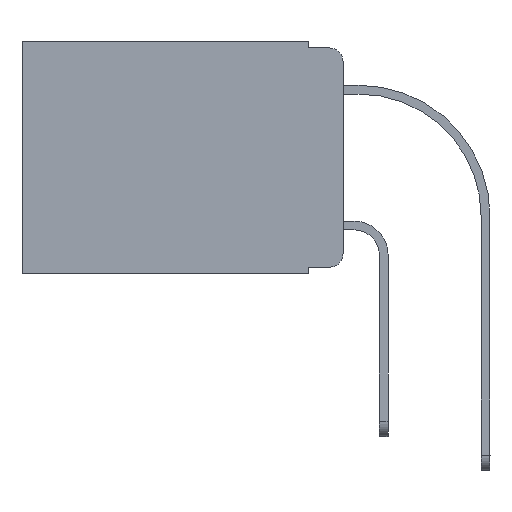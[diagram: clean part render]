
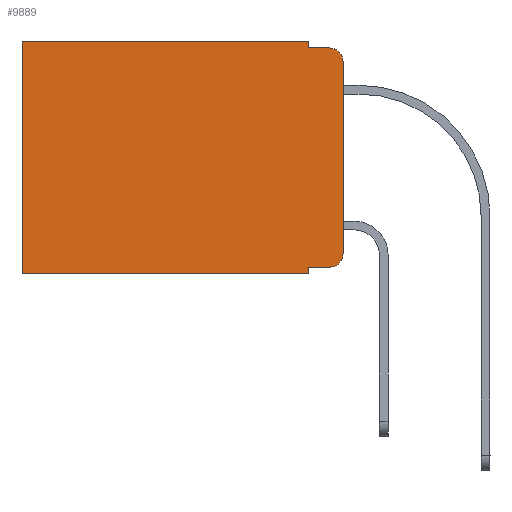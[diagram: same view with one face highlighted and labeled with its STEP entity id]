
A CAD part, left-side view. The second image highlights one B-rep face of the part: STEP entity #9889.
In plain terms, the highlighted planar face has unit normal (-1, 0, 0).
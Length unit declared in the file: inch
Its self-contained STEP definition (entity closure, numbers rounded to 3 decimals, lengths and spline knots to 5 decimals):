
#12 = CIRCLE ( 'NONE', #15573, 0.02 ) ;
#276 = ORIENTED_EDGE ( 'NONE', *, *, #1534, .F. ) ;
#453 = ORIENTED_EDGE ( 'NONE', *, *, #14678, .F. ) ;
#655 = CARTESIAN_POINT ( 'NONE',  ( 0.298, 0.02, -0.03 ) ) ;
#703 = VERTEX_POINT ( 'NONE', #19091 ) ;
#800 = DIRECTION ( 'NONE',  ( -1., 0., 0. ) ) ;
#911 = CARTESIAN_POINT ( 'NONE',  ( 0.298, 0., 0. ) ) ;
#935 = CARTESIAN_POINT ( 'NONE',  ( 0.298, 0.051, 0. ) ) ;
#1233 = DIRECTION ( 'NONE',  ( 1., 0., 0. ) ) ;
#1250 = LINE ( 'NONE', #10990, #7418 ) ;
#1534 = EDGE_CURVE ( 'NONE', #19817, #13339, #12464, .T. ) ;
#2334 = DIRECTION ( 'NONE',  ( 0., 0., -1. ) ) ;
#2341 = ORIENTED_EDGE ( 'NONE', *, *, #10339, .T. ) ;
#2630 = DIRECTION ( 'NONE',  ( 0., 0., -1. ) ) ;
#3657 = ORIENTED_EDGE ( 'NONE', *, *, #18781, .F. ) ;
#3850 = ORIENTED_EDGE ( 'NONE', *, *, #15713, .T. ) ;
#4126 = VERTEX_POINT ( 'NONE', #8880 ) ;
#4248 = VERTEX_POINT ( 'NONE', #20828 ) ;
#5466 = CARTESIAN_POINT ( 'NONE',  ( 0.298, 0.051, -0.01 ) ) ;
#6257 = CARTESIAN_POINT ( 'NONE',  ( 0.298, 0.051, -0.01 ) ) ;
#6722 = EDGE_CURVE ( 'NONE', #4126, #6739, #8010, .T. ) ;
#6739 = VERTEX_POINT ( 'NONE', #15595 ) ;
#6804 = LINE ( 'NONE', #13262, #10517 ) ;
#6893 = CARTESIAN_POINT ( 'NONE',  ( 0.298, 0.051, -0.333 ) ) ;
#7125 = DIRECTION ( 'NONE',  ( -1., 0., 0. ) ) ;
#7368 = DIRECTION ( 'NONE',  ( 0., 1., 0. ) ) ;
#7418 = VECTOR ( 'NONE', #2630, 39.37008 ) ;
#8010 = CIRCLE ( 'NONE', #11378, 0.02 ) ;
#8128 = CARTESIAN_POINT ( 'NONE',  ( 0.298, 0.02, -0.333 ) ) ;
#8704 = EDGE_LOOP ( 'NONE', ( #453, #10495, #18752, #3657, #20559, #9937, #276, #16006, #3850, #2341 ) ) ;
#8880 = CARTESIAN_POINT ( 'NONE',  ( 0.298, 0., -0.03 ) ) ;
#8945 = CARTESIAN_POINT ( 'NONE',  ( 0.298, 0.02, -0.313 ) ) ;
#9062 = DIRECTION ( 'NONE',  ( 0., 0., -1. ) ) ;
#9746 = VERTEX_POINT ( 'NONE', #8128 ) ;
#9889 = ADVANCED_FACE ( 'NONE', ( #12550 ), #12346, .F. ) ;
#9937 = ORIENTED_EDGE ( 'NONE', *, *, #14060, .T. ) ;
#10339 = EDGE_CURVE ( 'NONE', #9746, #703, #12, .T. ) ;
#10361 = DIRECTION ( 'NONE',  ( 0., 0., -1. ) ) ;
#10495 = ORIENTED_EDGE ( 'NONE', *, *, #6722, .T. ) ;
#10517 = VECTOR ( 'NONE', #19412, 39.37008 ) ;
#10990 = CARTESIAN_POINT ( 'NONE',  ( 0.298, 0.051, 0. ) ) ;
#11378 = AXIS2_PLACEMENT_3D ( 'NONE', #655, #7125, #15162 ) ;
#12094 = CARTESIAN_POINT ( 'NONE',  ( 0.298, 0.473, 0. ) ) ;
#12346 = PLANE ( 'NONE',  #15876 ) ;
#12443 = CARTESIAN_POINT ( 'NONE',  ( 0.298, 0., 0. ) ) ;
#12464 = LINE ( 'NONE', #18822, #20002 ) ;
#12506 = LINE ( 'NONE', #18974, #13254 ) ;
#12550 = FACE_OUTER_BOUND ( 'NONE', #8704, .T. ) ;
#13218 = CARTESIAN_POINT ( 'NONE',  ( 0.298, 0.051, -0.343 ) ) ;
#13254 = VECTOR ( 'NONE', #20872, 39.37008 ) ;
#13262 = CARTESIAN_POINT ( 'NONE',  ( 0.298, 0.473, 0. ) ) ;
#13339 = VERTEX_POINT ( 'NONE', #18342 ) ;
#13428 = LINE ( 'NONE', #935, #14182 ) ;
#13573 = VERTEX_POINT ( 'NONE', #6257 ) ;
#14060 = EDGE_CURVE ( 'NONE', #15548, #13339, #6804, .T. ) ;
#14182 = VECTOR ( 'NONE', #10361, 39.37008 ) ;
#14678 = EDGE_CURVE ( 'NONE', #4126, #703, #19898, .T. ) ;
#14985 = DIRECTION ( 'NONE',  ( 0., -1., 0. ) ) ;
#15162 = DIRECTION ( 'NONE',  ( 0., 0., -1. ) ) ;
#15276 = VECTOR ( 'NONE', #14985, 39.37008 ) ;
#15420 = LINE ( 'NONE', #911, #19944 ) ;
#15548 = VERTEX_POINT ( 'NONE', #12094 ) ;
#15573 = AXIS2_PLACEMENT_3D ( 'NONE', #8945, #800, #19162 ) ;
#15595 = CARTESIAN_POINT ( 'NONE',  ( 0.298, 0.02, -0.01 ) ) ;
#15713 = EDGE_CURVE ( 'NONE', #15823, #9746, #12506, .T. ) ;
#15823 = VERTEX_POINT ( 'NONE', #6893 ) ;
#15876 = AXIS2_PLACEMENT_3D ( 'NONE', #12443, #1233, #9062 ) ;
#16006 = ORIENTED_EDGE ( 'NONE', *, *, #17692, .F. ) ;
#16268 = VECTOR ( 'NONE', #2334, 39.37008 ) ;
#17692 = EDGE_CURVE ( 'NONE', #15823, #19817, #13428, .T. ) ;
#18342 = CARTESIAN_POINT ( 'NONE',  ( 0.298, 0.473, -0.343 ) ) ;
#18752 = ORIENTED_EDGE ( 'NONE', *, *, #18909, .F. ) ;
#18781 = EDGE_CURVE ( 'NONE', #4248, #13573, #1250, .T. ) ;
#18822 = CARTESIAN_POINT ( 'NONE',  ( 0.298, 0., -0.343 ) ) ;
#18909 = EDGE_CURVE ( 'NONE', #13573, #6739, #19943, .T. ) ;
#18974 = CARTESIAN_POINT ( 'NONE',  ( 0.298, 0.051, -0.333 ) ) ;
#19091 = CARTESIAN_POINT ( 'NONE',  ( 0.298, 0., -0.313 ) ) ;
#19162 = DIRECTION ( 'NONE',  ( 0., 0., -1. ) ) ;
#19307 = EDGE_CURVE ( 'NONE', #4248, #15548, #15420, .T. ) ;
#19412 = DIRECTION ( 'NONE',  ( 0., 0., -1. ) ) ;
#19817 = VERTEX_POINT ( 'NONE', #13218 ) ;
#19898 = LINE ( 'NONE', #20224, #16268 ) ;
#19943 = LINE ( 'NONE', #5466, #15276 ) ;
#19944 = VECTOR ( 'NONE', #7368, 39.37008 ) ;
#20002 = VECTOR ( 'NONE', #20428, 39.37008 ) ;
#20224 = CARTESIAN_POINT ( 'NONE',  ( 0.298, 0., 0. ) ) ;
#20428 = DIRECTION ( 'NONE',  ( 0., 1., 0. ) ) ;
#20559 = ORIENTED_EDGE ( 'NONE', *, *, #19307, .T. ) ;
#20828 = CARTESIAN_POINT ( 'NONE',  ( 0.298, 0.051, 0. ) ) ;
#20872 = DIRECTION ( 'NONE',  ( 0., -1., 0. ) ) ;
